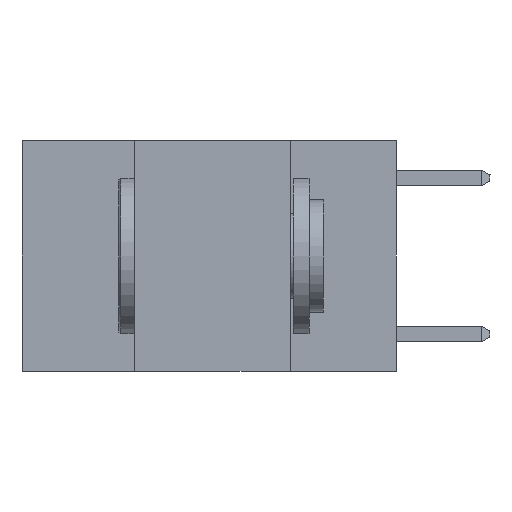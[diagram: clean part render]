
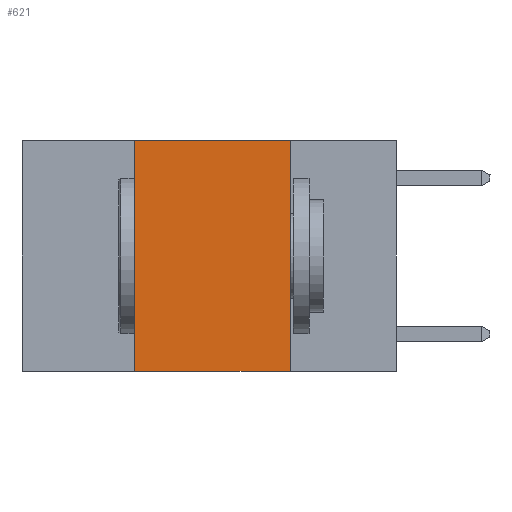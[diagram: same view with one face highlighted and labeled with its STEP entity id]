
A CAD part, left-side view. The second image highlights one B-rep face of the part: STEP entity #621.
In plain terms, the highlighted planar face has unit normal (-1, 0, 0).
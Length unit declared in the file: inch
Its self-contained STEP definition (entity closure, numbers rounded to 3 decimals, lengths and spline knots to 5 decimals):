
#33 = LINE ( 'NONE', #12184, #10731 ) ;
#500 = VERTEX_POINT ( 'NONE', #10020 ) ;
#532 = VERTEX_POINT ( 'NONE', #12077 ) ;
#621 = ADVANCED_FACE ( 'NONE', ( #5406 ), #8368, .F. ) ;
#662 = EDGE_CURVE ( 'NONE', #500, #10316, #6339, .T. ) ;
#1514 = CARTESIAN_POINT ( 'NONE',  ( 0., 0.42, 0. ) ) ;
#1634 = EDGE_CURVE ( 'NONE', #500, #11438, #4358, .T. ) ;
#2236 = CARTESIAN_POINT ( 'NONE',  ( 0., 0.42, 0. ) ) ;
#2354 = VECTOR ( 'NONE', #8384, 39.37008 ) ;
#4267 = CARTESIAN_POINT ( 'NONE',  ( 0., 0.6, -0.37 ) ) ;
#4358 = LINE ( 'NONE', #1514, #2354 ) ;
#4864 = VECTOR ( 'NONE', #8300, 39.37008 ) ;
#5406 = FACE_OUTER_BOUND ( 'NONE', #12229, .T. ) ;
#5539 = DIRECTION ( 'NONE',  ( 0., 0., -1. ) ) ;
#6339 = LINE ( 'NONE', #4267, #4864 ) ;
#6696 = ORIENTED_EDGE ( 'NONE', *, *, #10588, .F. ) ;
#6721 = EDGE_CURVE ( 'NONE', #532, #10316, #10601, .T. ) ;
#7499 = VECTOR ( 'NONE', #11719, 39.37008 ) ;
#8223 = DIRECTION ( 'NONE',  ( 0., -1., 0. ) ) ;
#8300 = DIRECTION ( 'NONE',  ( 0., -1., 0. ) ) ;
#8368 = PLANE ( 'NONE',  #9727 ) ;
#8384 = DIRECTION ( 'NONE',  ( 0., 0., 1. ) ) ;
#8498 = CARTESIAN_POINT ( 'NONE',  ( 0., 0.17, -0.37 ) ) ;
#9292 = DIRECTION ( 'NONE',  ( 1., 0., 0. ) ) ;
#9426 = CARTESIAN_POINT ( 'NONE',  ( 0., 0.6, 0. ) ) ;
#9727 = AXIS2_PLACEMENT_3D ( 'NONE', #9426, #9292, #5539 ) ;
#10020 = CARTESIAN_POINT ( 'NONE',  ( 0., 0.42, -0.37 ) ) ;
#10316 = VERTEX_POINT ( 'NONE', #8498 ) ;
#10588 = EDGE_CURVE ( 'NONE', #11438, #532, #33, .T. ) ;
#10601 = LINE ( 'NONE', #11847, #7499 ) ;
#10638 = ORIENTED_EDGE ( 'NONE', *, *, #1634, .F. ) ;
#10731 = VECTOR ( 'NONE', #8223, 39.37008 ) ;
#11358 = ORIENTED_EDGE ( 'NONE', *, *, #6721, .F. ) ;
#11438 = VERTEX_POINT ( 'NONE', #2236 ) ;
#11719 = DIRECTION ( 'NONE',  ( 0., 0., -1. ) ) ;
#11847 = CARTESIAN_POINT ( 'NONE',  ( 0., 0.17, 0. ) ) ;
#12077 = CARTESIAN_POINT ( 'NONE',  ( 0., 0.17, 0. ) ) ;
#12184 = CARTESIAN_POINT ( 'NONE',  ( 0., 0.6, 0. ) ) ;
#12229 = EDGE_LOOP ( 'NONE', ( #11358, #6696, #10638, #12785 ) ) ;
#12785 = ORIENTED_EDGE ( 'NONE', *, *, #662, .T. ) ;
